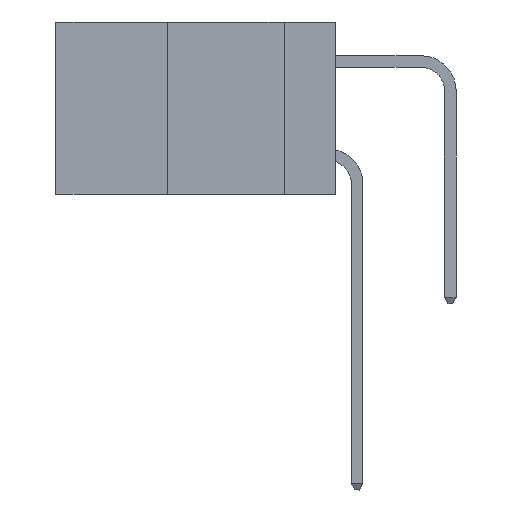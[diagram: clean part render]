
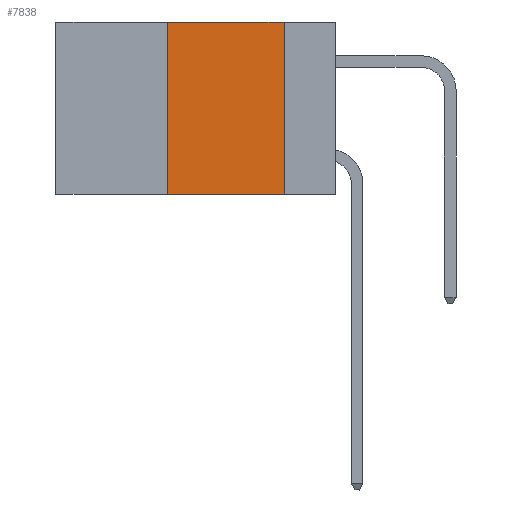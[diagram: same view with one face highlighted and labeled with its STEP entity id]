
A CAD part, left-side view. The second image highlights one B-rep face of the part: STEP entity #7838.
In plain terms, the highlighted planar face has unit normal (-1, 0, 0).
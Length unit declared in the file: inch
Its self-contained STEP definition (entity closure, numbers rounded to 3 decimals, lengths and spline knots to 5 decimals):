
#156 = CARTESIAN_POINT ( 'NONE',  ( 0., 0.11, 0. ) ) ;
#698 = ORIENTED_EDGE ( 'NONE', *, *, #8228, .F. ) ;
#716 = EDGE_CURVE ( 'NONE', #12664, #1968, #9349, .T. ) ;
#721 = LINE ( 'NONE', #9638, #2197 ) ;
#901 = DIRECTION ( 'NONE',  ( 1., 0., 0. ) ) ;
#1735 = LINE ( 'NONE', #156, #6757 ) ;
#1858 = EDGE_LOOP ( 'NONE', ( #698, #8264, #5340, #8829 ) ) ;
#1886 = PLANE ( 'NONE',  #1912 ) ;
#1912 = AXIS2_PLACEMENT_3D ( 'NONE', #9943, #901, #13012 ) ;
#1968 = VERTEX_POINT ( 'NONE', #11085 ) ;
#2160 = CARTESIAN_POINT ( 'NONE',  ( 0., 0.36, 0. ) ) ;
#2197 = VECTOR ( 'NONE', #3701, 39.37008 ) ;
#2663 = EDGE_CURVE ( 'NONE', #10844, #4697, #721, .T. ) ;
#3133 = DIRECTION ( 'NONE',  ( 0., 0., -1. ) ) ;
#3421 = LINE ( 'NONE', #2160, #10749 ) ;
#3701 = DIRECTION ( 'NONE',  ( 0., -1., 0. ) ) ;
#4697 = VERTEX_POINT ( 'NONE', #9697 ) ;
#5340 = ORIENTED_EDGE ( 'NONE', *, *, #7492, .F. ) ;
#6757 = VECTOR ( 'NONE', #3133, 39.37008 ) ;
#7407 = DIRECTION ( 'NONE',  ( 0., -1., 0. ) ) ;
#7492 = EDGE_CURVE ( 'NONE', #10844, #12664, #3421, .T. ) ;
#7641 = CARTESIAN_POINT ( 'NONE',  ( 0., 0.36, -0.37 ) ) ;
#7838 = ADVANCED_FACE ( 'NONE', ( #10946 ), #1886, .F. ) ;
#8228 = EDGE_CURVE ( 'NONE', #1968, #4697, #1735, .T. ) ;
#8264 = ORIENTED_EDGE ( 'NONE', *, *, #716, .F. ) ;
#8358 = CARTESIAN_POINT ( 'NONE',  ( 0., 0.36, 0. ) ) ;
#8460 = VECTOR ( 'NONE', #7407, 39.37008 ) ;
#8829 = ORIENTED_EDGE ( 'NONE', *, *, #2663, .T. ) ;
#9349 = LINE ( 'NONE', #11388, #8460 ) ;
#9638 = CARTESIAN_POINT ( 'NONE',  ( 0., 0.6, -0.37 ) ) ;
#9697 = CARTESIAN_POINT ( 'NONE',  ( 0., 0.11, -0.37 ) ) ;
#9943 = CARTESIAN_POINT ( 'NONE',  ( 0., 0.6, 0. ) ) ;
#10749 = VECTOR ( 'NONE', #12261, 39.37008 ) ;
#10844 = VERTEX_POINT ( 'NONE', #7641 ) ;
#10946 = FACE_OUTER_BOUND ( 'NONE', #1858, .T. ) ;
#11085 = CARTESIAN_POINT ( 'NONE',  ( 0., 0.11, 0. ) ) ;
#11388 = CARTESIAN_POINT ( 'NONE',  ( 0., 0.6, 0. ) ) ;
#12261 = DIRECTION ( 'NONE',  ( 0., 0., 1. ) ) ;
#12664 = VERTEX_POINT ( 'NONE', #8358 ) ;
#13012 = DIRECTION ( 'NONE',  ( 0., 0., -1. ) ) ;
